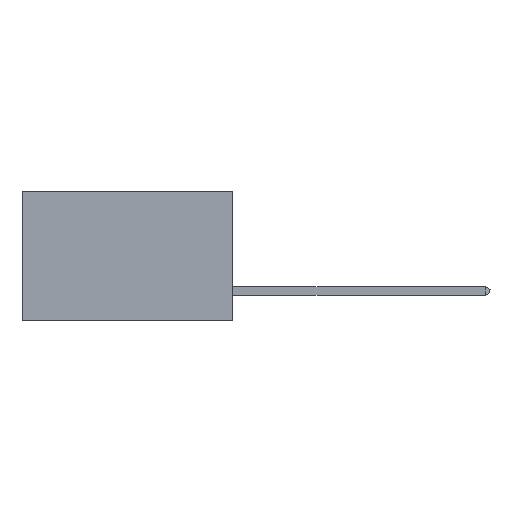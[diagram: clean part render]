
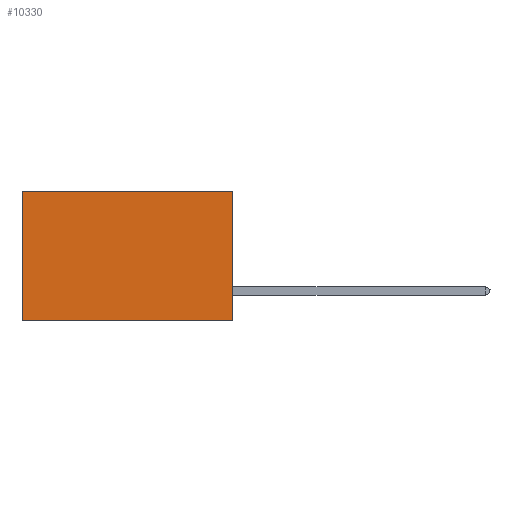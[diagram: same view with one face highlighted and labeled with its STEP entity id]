
A CAD part, left-side view. The second image highlights one B-rep face of the part: STEP entity #10330.
In plain terms, the highlighted planar face has unit normal (-1, 0, 0).
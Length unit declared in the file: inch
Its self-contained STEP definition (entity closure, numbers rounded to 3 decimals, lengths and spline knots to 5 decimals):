
#75 = EDGE_LOOP ( 'NONE', ( #20088, #30326, #14779, #17288 ) ) ;
#1604 = CARTESIAN_POINT ( 'NONE',  ( 0.2875, 0.6, 0. ) ) ;
#2860 = VECTOR ( 'NONE', #11091, 39.37008 ) ;
#3675 = LINE ( 'NONE', #18547, #2860 ) ;
#4726 = CARTESIAN_POINT ( 'NONE',  ( 0.2875, 0., 0. ) ) ;
#4755 = VERTEX_POINT ( 'NONE', #31242 ) ;
#5554 = LINE ( 'NONE', #21940, #30846 ) ;
#6622 = DIRECTION ( 'NONE',  ( 0., 0., -1. ) ) ;
#8873 = VERTEX_POINT ( 'NONE', #1604 ) ;
#9293 = CARTESIAN_POINT ( 'NONE',  ( 0.2875, 0., 0. ) ) ;
#10054 = PLANE ( 'NONE',  #22009 ) ;
#10330 = ADVANCED_FACE ( 'NONE', ( #11642 ), #10054, .F. ) ;
#10962 = VECTOR ( 'NONE', #6622, 39.37008 ) ;
#11091 = DIRECTION ( 'NONE',  ( 0., 1., 0. ) ) ;
#11466 = EDGE_CURVE ( 'NONE', #8873, #4755, #5554, .T. ) ;
#11642 = FACE_OUTER_BOUND ( 'NONE', #75, .T. ) ;
#12001 = LINE ( 'NONE', #30921, #18453 ) ;
#12200 = DIRECTION ( 'NONE',  ( 0., 0., -1. ) ) ;
#13090 = VERTEX_POINT ( 'NONE', #25743 ) ;
#14065 = DIRECTION ( 'NONE',  ( 0., 1., 0. ) ) ;
#14779 = ORIENTED_EDGE ( 'NONE', *, *, #28968, .F. ) ;
#16360 = EDGE_CURVE ( 'NONE', #13090, #8873, #3675, .T. ) ;
#16994 = LINE ( 'NONE', #9293, #10962 ) ;
#17288 = ORIENTED_EDGE ( 'NONE', *, *, #16360, .T. ) ;
#18453 = VECTOR ( 'NONE', #14065, 39.37008 ) ;
#18547 = CARTESIAN_POINT ( 'NONE',  ( 0.2875, 0., 0. ) ) ;
#19728 = CARTESIAN_POINT ( 'NONE',  ( 0.2875, 0., -0.37 ) ) ;
#20088 = ORIENTED_EDGE ( 'NONE', *, *, #11466, .T. ) ;
#21940 = CARTESIAN_POINT ( 'NONE',  ( 0.2875, 0.6, 0. ) ) ;
#22009 = AXIS2_PLACEMENT_3D ( 'NONE', #4726, #25611, #12200 ) ;
#22047 = DIRECTION ( 'NONE',  ( 0., 0., -1. ) ) ;
#22988 = VERTEX_POINT ( 'NONE', #19728 ) ;
#25611 = DIRECTION ( 'NONE',  ( 1., 0., 0. ) ) ;
#25743 = CARTESIAN_POINT ( 'NONE',  ( 0.2875, 0., 0. ) ) ;
#28968 = EDGE_CURVE ( 'NONE', #13090, #22988, #16994, .T. ) ;
#30326 = ORIENTED_EDGE ( 'NONE', *, *, #31187, .F. ) ;
#30846 = VECTOR ( 'NONE', #22047, 39.37008 ) ;
#30921 = CARTESIAN_POINT ( 'NONE',  ( 0.2875, 0., -0.37 ) ) ;
#31187 = EDGE_CURVE ( 'NONE', #22988, #4755, #12001, .T. ) ;
#31242 = CARTESIAN_POINT ( 'NONE',  ( 0.2875, 0.6, -0.37 ) ) ;
